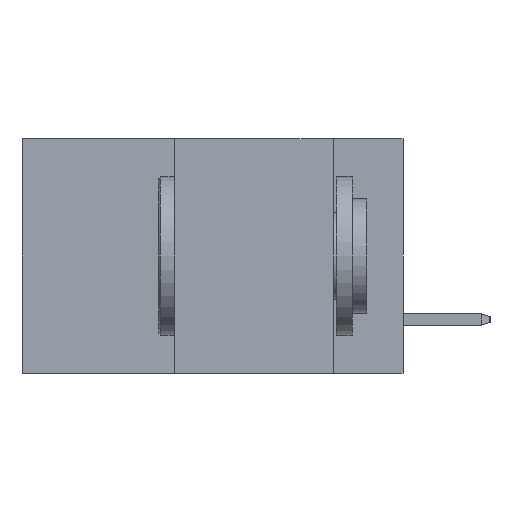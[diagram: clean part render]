
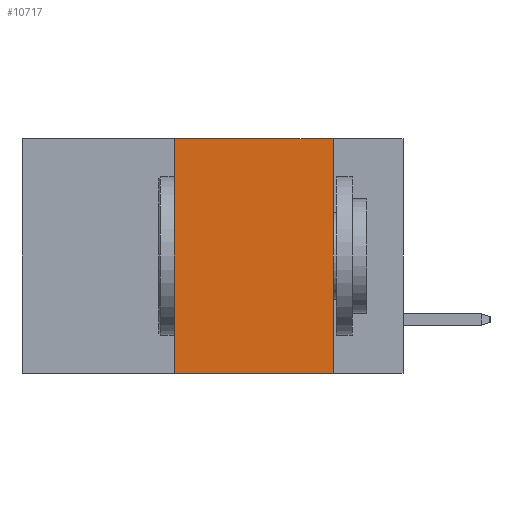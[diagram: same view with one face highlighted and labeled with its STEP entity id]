
A CAD part, left-side view. The second image highlights one B-rep face of the part: STEP entity #10717.
In plain terms, the highlighted planar face has unit normal (-1, 0, 0).
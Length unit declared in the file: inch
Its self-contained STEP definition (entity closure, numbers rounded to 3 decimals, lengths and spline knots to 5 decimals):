
#76 = DIRECTION ( 'NONE',  ( 0., -1., 0. ) ) ;
#160 = CARTESIAN_POINT ( 'NONE',  ( 0., 0.6, -0.37 ) ) ;
#455 = CARTESIAN_POINT ( 'NONE',  ( 0., 0.36, 0. ) ) ;
#1106 = CARTESIAN_POINT ( 'NONE',  ( 0., 0.36, 0. ) ) ;
#1506 = LINE ( 'NONE', #5577, #3677 ) ;
#1837 = LINE ( 'NONE', #455, #6838 ) ;
#2062 = VECTOR ( 'NONE', #76, 39.37008 ) ;
#2145 = CARTESIAN_POINT ( 'NONE',  ( 0., 0.11, -0.37 ) ) ;
#2536 = DIRECTION ( 'NONE',  ( 1., 0., 0. ) ) ;
#2649 = EDGE_CURVE ( 'NONE', #16465, #16978, #15173, .T. ) ;
#2663 = EDGE_CURVE ( 'NONE', #8385, #16978, #3848, .T. ) ;
#3162 = ORIENTED_EDGE ( 'NONE', *, *, #2663, .T. ) ;
#3677 = VECTOR ( 'NONE', #15828, 39.37008 ) ;
#3848 = LINE ( 'NONE', #160, #2062 ) ;
#5100 = CARTESIAN_POINT ( 'NONE',  ( 0., 0.11, 0. ) ) ;
#5262 = ORIENTED_EDGE ( 'NONE', *, *, #9175, .F. ) ;
#5577 = CARTESIAN_POINT ( 'NONE',  ( 0., 0.6, 0. ) ) ;
#5741 = DIRECTION ( 'NONE',  ( 0., 0., 1. ) ) ;
#6356 = DIRECTION ( 'NONE',  ( 0., 0., -1. ) ) ;
#6522 = FACE_OUTER_BOUND ( 'NONE', #10455, .T. ) ;
#6838 = VECTOR ( 'NONE', #5741, 39.37008 ) ;
#6960 = ORIENTED_EDGE ( 'NONE', *, *, #2649, .F. ) ;
#7212 = CARTESIAN_POINT ( 'NONE',  ( 0., 0.36, -0.37 ) ) ;
#8385 = VERTEX_POINT ( 'NONE', #7212 ) ;
#9175 = EDGE_CURVE ( 'NONE', #11540, #16465, #1506, .T. ) ;
#10072 = CARTESIAN_POINT ( 'NONE',  ( 0., 0.11, 0. ) ) ;
#10136 = ORIENTED_EDGE ( 'NONE', *, *, #13590, .F. ) ;
#10455 = EDGE_LOOP ( 'NONE', ( #6960, #5262, #10136, #3162 ) ) ;
#10717 = ADVANCED_FACE ( 'NONE', ( #6522 ), #15551, .F. ) ;
#11540 = VERTEX_POINT ( 'NONE', #1106 ) ;
#12839 = AXIS2_PLACEMENT_3D ( 'NONE', #15807, #2536, #6356 ) ;
#13590 = EDGE_CURVE ( 'NONE', #8385, #11540, #1837, .T. ) ;
#13650 = VECTOR ( 'NONE', #15247, 39.37008 ) ;
#15173 = LINE ( 'NONE', #10072, #13650 ) ;
#15247 = DIRECTION ( 'NONE',  ( 0., 0., -1. ) ) ;
#15551 = PLANE ( 'NONE',  #12839 ) ;
#15807 = CARTESIAN_POINT ( 'NONE',  ( 0., 0.6, 0. ) ) ;
#15828 = DIRECTION ( 'NONE',  ( 0., -1., 0. ) ) ;
#16465 = VERTEX_POINT ( 'NONE', #5100 ) ;
#16978 = VERTEX_POINT ( 'NONE', #2145 ) ;
